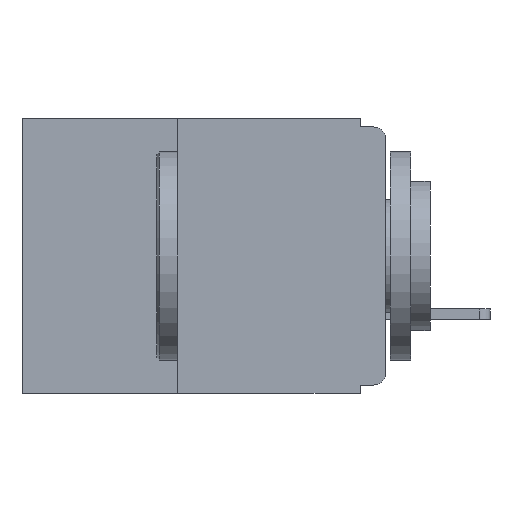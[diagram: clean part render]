
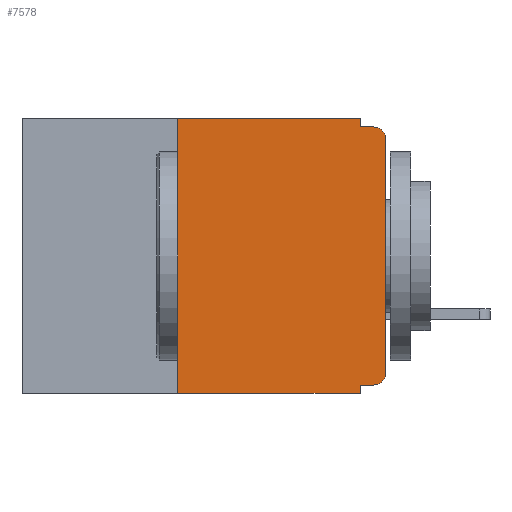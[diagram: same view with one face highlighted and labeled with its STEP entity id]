
A CAD part, left-side view. The second image highlights one B-rep face of the part: STEP entity #7578.
In plain terms, the highlighted planar face has unit normal (-1, 0, 0).
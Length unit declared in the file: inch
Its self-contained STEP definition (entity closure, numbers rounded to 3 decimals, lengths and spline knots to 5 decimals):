
#153 = ORIENTED_EDGE ( 'NONE', *, *, #13477, .F. ) ;
#391 = VERTEX_POINT ( 'NONE', #16525 ) ;
#412 = CIRCLE ( 'NONE', #8462, 0.015 ) ;
#606 = LINE ( 'NONE', #8044, #12628 ) ;
#684 = VERTEX_POINT ( 'NONE', #12703 ) ;
#693 = CARTESIAN_POINT ( 'NONE',  ( 0., 0.015, -0.305 ) ) ;
#842 = VECTOR ( 'NONE', #18012, 39.37008 ) ;
#1003 = LINE ( 'NONE', #19450, #8856 ) ;
#2003 = DIRECTION ( 'NONE',  ( 0., -1., 0. ) ) ;
#2158 = ORIENTED_EDGE ( 'NONE', *, *, #13233, .T. ) ;
#2288 = DIRECTION ( 'NONE',  ( 0., 0., -1. ) ) ;
#2401 = AXIS2_PLACEMENT_3D ( 'NONE', #9000, #19900, #10571 ) ;
#3328 = LINE ( 'NONE', #12948, #19389 ) ;
#3391 = CARTESIAN_POINT ( 'NONE',  ( 0., 0.015, -0.01 ) ) ;
#3605 = ORIENTED_EDGE ( 'NONE', *, *, #20151, .T. ) ;
#3837 = VERTEX_POINT ( 'NONE', #13712 ) ;
#4001 = DIRECTION ( 'NONE',  ( 0., 0., -1. ) ) ;
#4041 = EDGE_CURVE ( 'NONE', #18125, #19635, #606, .T. ) ;
#5434 = DIRECTION ( 'NONE',  ( 0., 0., -1. ) ) ;
#5517 = DIRECTION ( 'NONE',  ( 1., 0., 0. ) ) ;
#5542 = PLANE ( 'NONE',  #15475 ) ;
#5577 = CARTESIAN_POINT ( 'NONE',  ( 0., 0.031, 0. ) ) ;
#6050 = CARTESIAN_POINT ( 'NONE',  ( 0., 0.437, 0. ) ) ;
#6521 = ORIENTED_EDGE ( 'NONE', *, *, #17656, .F. ) ;
#7578 = ADVANCED_FACE ( 'NONE', ( #7803 ), #5542, .F. ) ;
#7686 = VERTEX_POINT ( 'NONE', #3391 ) ;
#7803 = FACE_OUTER_BOUND ( 'NONE', #12080, .T. ) ;
#7902 = DIRECTION ( 'NONE',  ( 0., 0., -1. ) ) ;
#8006 = EDGE_CURVE ( 'NONE', #15974, #19789, #412, .T. ) ;
#8044 = CARTESIAN_POINT ( 'NONE',  ( 0., 0.031, -0.33 ) ) ;
#8462 = AXIS2_PLACEMENT_3D ( 'NONE', #693, #11644, #2288 ) ;
#8856 = VECTOR ( 'NONE', #13282, 39.37008 ) ;
#8985 = LINE ( 'NONE', #10802, #16811 ) ;
#9000 = CARTESIAN_POINT ( 'NONE',  ( 0., 0.015, -0.025 ) ) ;
#9197 = LINE ( 'NONE', #16438, #842 ) ;
#9296 = EDGE_CURVE ( 'NONE', #11008, #19635, #12360, .T. ) ;
#9356 = LINE ( 'NONE', #16543, #12035 ) ;
#10316 = CARTESIAN_POINT ( 'NONE',  ( 0., 0.015, -0.32 ) ) ;
#10571 = DIRECTION ( 'NONE',  ( 0., 0., -1. ) ) ;
#10802 = CARTESIAN_POINT ( 'NONE',  ( 0., 0., -0.32 ) ) ;
#11008 = VERTEX_POINT ( 'NONE', #11055 ) ;
#11055 = CARTESIAN_POINT ( 'NONE',  ( 0., 0.25, -0.33 ) ) ;
#11493 = CARTESIAN_POINT ( 'NONE',  ( 0., 0.031, -0.32 ) ) ;
#11566 = VERTEX_POINT ( 'NONE', #18603 ) ;
#11644 = DIRECTION ( 'NONE',  ( -1., 0., 0. ) ) ;
#11785 = EDGE_CURVE ( 'NONE', #684, #7686, #3328, .T. ) ;
#11802 = ORIENTED_EDGE ( 'NONE', *, *, #11785, .F. ) ;
#12035 = VECTOR ( 'NONE', #18102, 39.37008 ) ;
#12047 = CARTESIAN_POINT ( 'NONE',  ( 0., 0.031, -0.33 ) ) ;
#12080 = EDGE_LOOP ( 'NONE', ( #3605, #2158, #11802, #6521, #19567, #153, #13411, #16330, #17170, #15654 ) ) ;
#12360 = LINE ( 'NONE', #13247, #18450 ) ;
#12378 = DIRECTION ( 'NONE',  ( 0., 1., 0. ) ) ;
#12628 = VECTOR ( 'NONE', #7902, 39.37008 ) ;
#12703 = CARTESIAN_POINT ( 'NONE',  ( 0., 0.031, -0.01 ) ) ;
#12948 = CARTESIAN_POINT ( 'NONE',  ( 0., 0., -0.01 ) ) ;
#13233 = EDGE_CURVE ( 'NONE', #3837, #7686, #18384, .T. ) ;
#13247 = CARTESIAN_POINT ( 'NONE',  ( 0., 0.437, -0.33 ) ) ;
#13282 = DIRECTION ( 'NONE',  ( 0., 0., 1. ) ) ;
#13411 = ORIENTED_EDGE ( 'NONE', *, *, #9296, .T. ) ;
#13477 = EDGE_CURVE ( 'NONE', #11008, #11566, #1003, .T. ) ;
#13564 = EDGE_CURVE ( 'NONE', #11566, #391, #9356, .T. ) ;
#13712 = CARTESIAN_POINT ( 'NONE',  ( 0., 0., -0.025 ) ) ;
#13947 = CARTESIAN_POINT ( 'NONE',  ( 0., 0., -0.305 ) ) ;
#15475 = AXIS2_PLACEMENT_3D ( 'NONE', #6050, #5517, #5434 ) ;
#15654 = ORIENTED_EDGE ( 'NONE', *, *, #8006, .T. ) ;
#15827 = LINE ( 'NONE', #5577, #19483 ) ;
#15974 = VERTEX_POINT ( 'NONE', #10316 ) ;
#16330 = ORIENTED_EDGE ( 'NONE', *, *, #4041, .F. ) ;
#16359 = DIRECTION ( 'NONE',  ( 0., -1., 0. ) ) ;
#16438 = CARTESIAN_POINT ( 'NONE',  ( 0., 0., 0. ) ) ;
#16525 = CARTESIAN_POINT ( 'NONE',  ( 0., 0.031, 0. ) ) ;
#16543 = CARTESIAN_POINT ( 'NONE',  ( 0., 0.437, 0. ) ) ;
#16811 = VECTOR ( 'NONE', #12378, 39.37008 ) ;
#17170 = ORIENTED_EDGE ( 'NONE', *, *, #18447, .F. ) ;
#17656 = EDGE_CURVE ( 'NONE', #391, #684, #15827, .T. ) ;
#18012 = DIRECTION ( 'NONE',  ( 0., 0., 1. ) ) ;
#18102 = DIRECTION ( 'NONE',  ( 0., -1., 0. ) ) ;
#18125 = VERTEX_POINT ( 'NONE', #11493 ) ;
#18384 = CIRCLE ( 'NONE', #2401, 0.015 ) ;
#18447 = EDGE_CURVE ( 'NONE', #15974, #18125, #8985, .T. ) ;
#18450 = VECTOR ( 'NONE', #16359, 39.37008 ) ;
#18603 = CARTESIAN_POINT ( 'NONE',  ( 0., 0.25, 0. ) ) ;
#19389 = VECTOR ( 'NONE', #2003, 39.37008 ) ;
#19450 = CARTESIAN_POINT ( 'NONE',  ( 0., 0.25, -0.33 ) ) ;
#19483 = VECTOR ( 'NONE', #4001, 39.37008 ) ;
#19567 = ORIENTED_EDGE ( 'NONE', *, *, #13564, .F. ) ;
#19635 = VERTEX_POINT ( 'NONE', #12047 ) ;
#19789 = VERTEX_POINT ( 'NONE', #13947 ) ;
#19900 = DIRECTION ( 'NONE',  ( -1., 0., 0. ) ) ;
#20151 = EDGE_CURVE ( 'NONE', #19789, #3837, #9197, .T. ) ;
